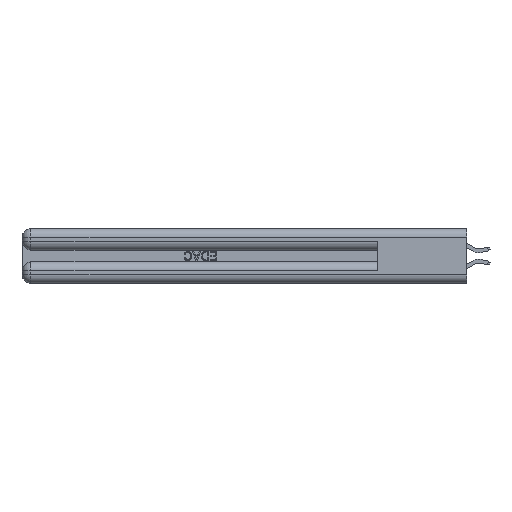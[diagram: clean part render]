
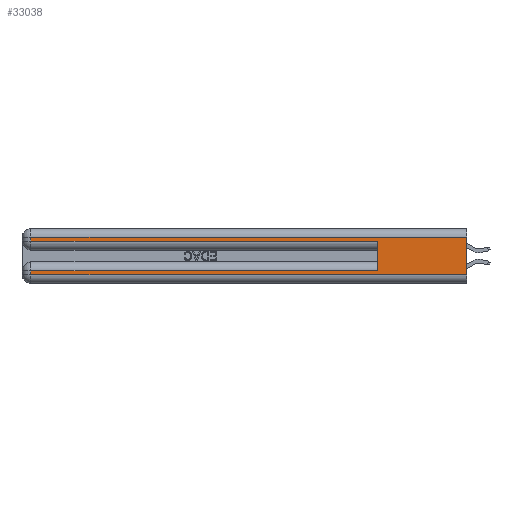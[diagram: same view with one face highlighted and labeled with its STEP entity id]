
A CAD part, left-side view. The second image highlights one B-rep face of the part: STEP entity #33038.
In plain terms, the highlighted planar face has unit normal (-1, 0, 0).
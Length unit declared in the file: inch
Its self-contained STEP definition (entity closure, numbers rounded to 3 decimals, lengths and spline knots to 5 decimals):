
#2154 = DIRECTION ( 'NONE',  ( 0., -1., 0. ) ) ;
#2438 = ORIENTED_EDGE ( 'NONE', *, *, #19770, .T. ) ;
#2776 = ORIENTED_EDGE ( 'NONE', *, *, #16429, .T. ) ;
#3169 = CARTESIAN_POINT ( 'NONE',  ( 0., 0., 0.37 ) ) ;
#3358 = VERTEX_POINT ( 'NONE', #42788 ) ;
#3595 = DIRECTION ( 'NONE',  ( 0., 0., -1. ) ) ;
#3608 = VECTOR ( 'NONE', #30763, 39.37008 ) ;
#4415 = LINE ( 'NONE', #9562, #5474 ) ;
#5474 = VECTOR ( 'NONE', #33063, 39.37008 ) ;
#6569 = DIRECTION ( 'NONE',  ( 1., 0., 0. ) ) ;
#7262 = CARTESIAN_POINT ( 'NONE',  ( 0., 0., 0.085 ) ) ;
#7693 = EDGE_CURVE ( 'NONE', #41238, #3358, #22925, .T. ) ;
#8136 = VERTEX_POINT ( 'NONE', #39875 ) ;
#8819 = VERTEX_POINT ( 'NONE', #17001 ) ;
#9562 = CARTESIAN_POINT ( 'NONE',  ( 0., 0.6, 0.145 ) ) ;
#12555 = EDGE_CURVE ( 'NONE', #33409, #33835, #30433, .T. ) ;
#12820 = DIRECTION ( 'NONE',  ( 0., 1., 0. ) ) ;
#14019 = VECTOR ( 'NONE', #22791, 39.37008 ) ;
#14401 = EDGE_LOOP ( 'NONE', ( #37359, #2776, #36358, #2438, #30582, #42963, #38342, #31454 ) ) ;
#15117 = CARTESIAN_POINT ( 'NONE',  ( 0., 0., 0.06 ) ) ;
#15929 = CARTESIAN_POINT ( 'NONE',  ( 0., 0., 0.06 ) ) ;
#16016 = LINE ( 'NONE', #19051, #22770 ) ;
#16254 = CARTESIAN_POINT ( 'NONE',  ( 0., 0., 0.31 ) ) ;
#16429 = EDGE_CURVE ( 'NONE', #8136, #41238, #25896, .T. ) ;
#16539 = FACE_OUTER_BOUND ( 'NONE', #14401, .T. ) ;
#17001 = CARTESIAN_POINT ( 'NONE',  ( 0., 2.94, 0.06 ) ) ;
#19051 = CARTESIAN_POINT ( 'NONE',  ( 0., 0., 0.285 ) ) ;
#19640 = CARTESIAN_POINT ( 'NONE',  ( 0., 0., 0.37 ) ) ;
#19770 = EDGE_CURVE ( 'NONE', #3358, #24085, #16016, .T. ) ;
#19860 = LINE ( 'NONE', #15929, #36630 ) ;
#20156 = DIRECTION ( 'NONE',  ( 0., 0., -1. ) ) ;
#20838 = VERTEX_POINT ( 'NONE', #15117 ) ;
#22770 = VECTOR ( 'NONE', #2154, 39.37008 ) ;
#22791 = DIRECTION ( 'NONE',  ( 0., 0., -1. ) ) ;
#22925 = LINE ( 'NONE', #23740, #33957 ) ;
#23056 = VECTOR ( 'NONE', #20156, 39.37008 ) ;
#23319 = PLANE ( 'NONE',  #26349 ) ;
#23740 = CARTESIAN_POINT ( 'NONE',  ( 0., 2.94, 0.37 ) ) ;
#24085 = VERTEX_POINT ( 'NONE', #42514 ) ;
#25500 = CARTESIAN_POINT ( 'NONE',  ( 0., 0.6, 0.085 ) ) ;
#25896 = LINE ( 'NONE', #16254, #33788 ) ;
#26127 = EDGE_CURVE ( 'NONE', #8136, #20838, #32921, .T. ) ;
#26349 = AXIS2_PLACEMENT_3D ( 'NONE', #3169, #6569, #30075 ) ;
#26697 = CARTESIAN_POINT ( 'NONE',  ( 0., 2.94, 0.37 ) ) ;
#29226 = DIRECTION ( 'NONE',  ( 0., -1., 0. ) ) ;
#29536 = EDGE_CURVE ( 'NONE', #33835, #8819, #42974, .T. ) ;
#30075 = DIRECTION ( 'NONE',  ( 0., 0., -1. ) ) ;
#30433 = LINE ( 'NONE', #7262, #3608 ) ;
#30582 = ORIENTED_EDGE ( 'NONE', *, *, #38336, .F. ) ;
#30763 = DIRECTION ( 'NONE',  ( 0., 1., 0. ) ) ;
#30983 = EDGE_CURVE ( 'NONE', #8819, #20838, #19860, .T. ) ;
#31454 = ORIENTED_EDGE ( 'NONE', *, *, #30983, .T. ) ;
#32921 = LINE ( 'NONE', #19640, #14019 ) ;
#33038 = ADVANCED_FACE ( 'NONE', ( #16539 ), #23319, .F. ) ;
#33063 = DIRECTION ( 'NONE',  ( 0., 0., 1. ) ) ;
#33308 = CARTESIAN_POINT ( 'NONE',  ( 0., 2.94, 0.085 ) ) ;
#33409 = VERTEX_POINT ( 'NONE', #25500 ) ;
#33788 = VECTOR ( 'NONE', #12820, 39.37008 ) ;
#33835 = VERTEX_POINT ( 'NONE', #33308 ) ;
#33957 = VECTOR ( 'NONE', #3595, 39.37008 ) ;
#36358 = ORIENTED_EDGE ( 'NONE', *, *, #7693, .T. ) ;
#36630 = VECTOR ( 'NONE', #29226, 39.37008 ) ;
#37359 = ORIENTED_EDGE ( 'NONE', *, *, #26127, .F. ) ;
#38336 = EDGE_CURVE ( 'NONE', #33409, #24085, #4415, .T. ) ;
#38342 = ORIENTED_EDGE ( 'NONE', *, *, #29536, .T. ) ;
#39875 = CARTESIAN_POINT ( 'NONE',  ( 0., 0., 0.31 ) ) ;
#41238 = VERTEX_POINT ( 'NONE', #42783 ) ;
#42514 = CARTESIAN_POINT ( 'NONE',  ( 0., 0.6, 0.285 ) ) ;
#42783 = CARTESIAN_POINT ( 'NONE',  ( 0., 2.94, 0.31 ) ) ;
#42788 = CARTESIAN_POINT ( 'NONE',  ( 0., 2.94, 0.285 ) ) ;
#42963 = ORIENTED_EDGE ( 'NONE', *, *, #12555, .T. ) ;
#42974 = LINE ( 'NONE', #26697, #23056 ) ;
